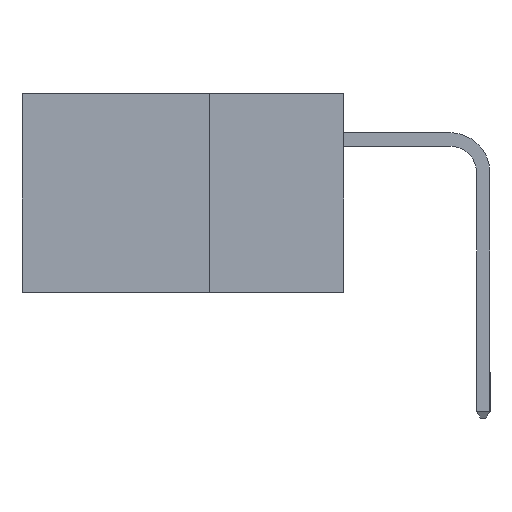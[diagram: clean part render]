
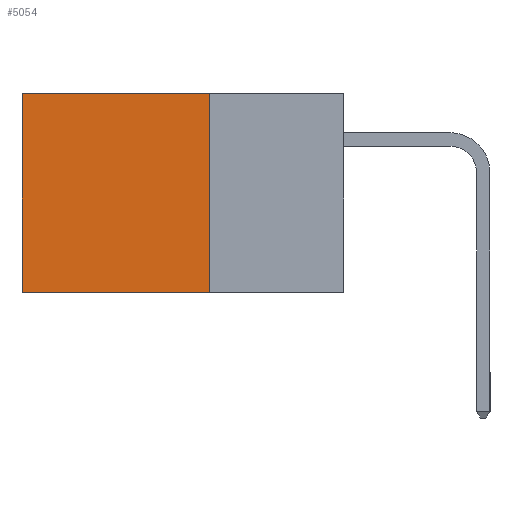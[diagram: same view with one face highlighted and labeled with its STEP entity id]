
A CAD part, left-side view. The second image highlights one B-rep face of the part: STEP entity #5054.
In plain terms, the highlighted planar face has unit normal (-1, 0, 0).
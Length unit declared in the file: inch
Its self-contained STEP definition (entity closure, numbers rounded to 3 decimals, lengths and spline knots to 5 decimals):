
#405 = CARTESIAN_POINT ( 'NONE',  ( 0.298, 0.6, 0. ) ) ;
#845 = EDGE_CURVE ( 'NONE', #14714, #14268, #12630, .T. ) ;
#2924 = CARTESIAN_POINT ( 'NONE',  ( 0.298, 0.25, -0.37 ) ) ;
#2966 = CARTESIAN_POINT ( 'NONE',  ( 0.298, 0.6, 0. ) ) ;
#4253 = DIRECTION ( 'NONE',  ( 0., 1., 0. ) ) ;
#4287 = VECTOR ( 'NONE', #12785, 39.37008 ) ;
#4400 = ORIENTED_EDGE ( 'NONE', *, *, #9657, .F. ) ;
#5054 = ADVANCED_FACE ( 'NONE', ( #18372 ), #21273, .F. ) ;
#5166 = ORIENTED_EDGE ( 'NONE', *, *, #8569, .F. ) ;
#5751 = CARTESIAN_POINT ( 'NONE',  ( 0.298, 0.6, -0.37 ) ) ;
#8112 = DIRECTION ( 'NONE',  ( 0., 1., 0. ) ) ;
#8297 = DIRECTION ( 'NONE',  ( 0., 0., -1. ) ) ;
#8569 = EDGE_CURVE ( 'NONE', #19727, #19377, #9069, .T. ) ;
#9069 = LINE ( 'NONE', #19537, #4287 ) ;
#9589 = VECTOR ( 'NONE', #8112, 39.37008 ) ;
#9657 = EDGE_CURVE ( 'NONE', #19377, #14268, #18663, .T. ) ;
#10149 = ORIENTED_EDGE ( 'NONE', *, *, #845, .T. ) ;
#10481 = VECTOR ( 'NONE', #8297, 39.37008 ) ;
#10669 = LINE ( 'NONE', #18381, #21308 ) ;
#11120 = CARTESIAN_POINT ( 'NONE',  ( 0.298, 0.25, 0. ) ) ;
#12630 = LINE ( 'NONE', #2966, #10481 ) ;
#12785 = DIRECTION ( 'NONE',  ( 0., 0., -1. ) ) ;
#13767 = ORIENTED_EDGE ( 'NONE', *, *, #20112, .T. ) ;
#14268 = VERTEX_POINT ( 'NONE', #5751 ) ;
#14714 = VERTEX_POINT ( 'NONE', #405 ) ;
#15951 = AXIS2_PLACEMENT_3D ( 'NONE', #11120, #19516, #16380 ) ;
#15962 = CARTESIAN_POINT ( 'NONE',  ( 0.298, 0.25, -0.37 ) ) ;
#16380 = DIRECTION ( 'NONE',  ( 0., 0., -1. ) ) ;
#17116 = EDGE_LOOP ( 'NONE', ( #10149, #4400, #5166, #13767 ) ) ;
#18372 = FACE_OUTER_BOUND ( 'NONE', #17116, .T. ) ;
#18381 = CARTESIAN_POINT ( 'NONE',  ( 0.298, 0.25, 0. ) ) ;
#18663 = LINE ( 'NONE', #2924, #9589 ) ;
#19377 = VERTEX_POINT ( 'NONE', #15962 ) ;
#19516 = DIRECTION ( 'NONE',  ( 1., 0., 0. ) ) ;
#19537 = CARTESIAN_POINT ( 'NONE',  ( 0.298, 0.25, 0. ) ) ;
#19727 = VERTEX_POINT ( 'NONE', #22025 ) ;
#20112 = EDGE_CURVE ( 'NONE', #19727, #14714, #10669, .T. ) ;
#21273 = PLANE ( 'NONE',  #15951 ) ;
#21308 = VECTOR ( 'NONE', #4253, 39.37008 ) ;
#22025 = CARTESIAN_POINT ( 'NONE',  ( 0.298, 0.25, 0. ) ) ;
